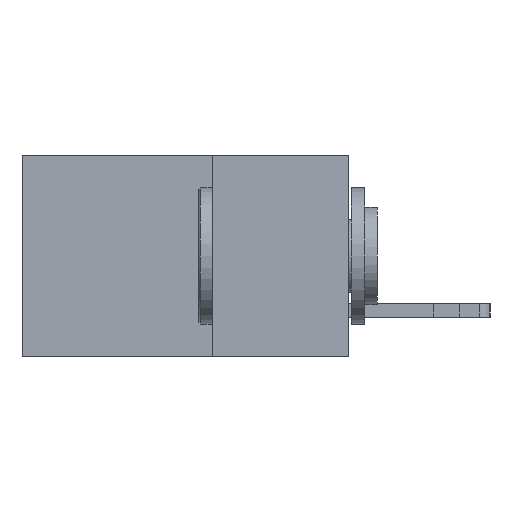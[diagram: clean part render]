
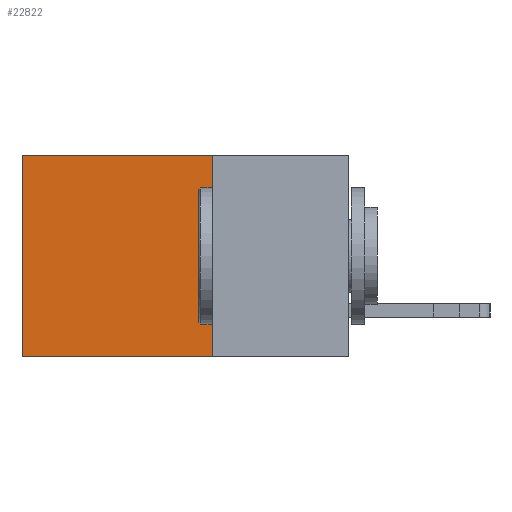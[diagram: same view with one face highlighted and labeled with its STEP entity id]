
A CAD part, left-side view. The second image highlights one B-rep face of the part: STEP entity #22822.
In plain terms, the highlighted planar face has unit normal (-1, 0, 0).
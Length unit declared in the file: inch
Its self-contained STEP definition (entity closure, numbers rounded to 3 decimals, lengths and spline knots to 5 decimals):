
#579 = CARTESIAN_POINT ( 'NONE',  ( 0.298, 0.6, 0. ) ) ;
#1082 = VERTEX_POINT ( 'NONE', #18681 ) ;
#2057 = CARTESIAN_POINT ( 'NONE',  ( 0.298, 0.25, 0. ) ) ;
#2313 = EDGE_CURVE ( 'NONE', #15424, #1082, #12239, .T. ) ;
#3681 = CARTESIAN_POINT ( 'NONE',  ( 0.298, 0.6, 0. ) ) ;
#4080 = DIRECTION ( 'NONE',  ( 1., 0., 0. ) ) ;
#4758 = CARTESIAN_POINT ( 'NONE',  ( 0.298, 0.25, 0. ) ) ;
#5892 = EDGE_CURVE ( 'NONE', #13069, #15424, #20276, .T. ) ;
#6371 = ORIENTED_EDGE ( 'NONE', *, *, #23649, .T. ) ;
#7749 = CARTESIAN_POINT ( 'NONE',  ( 0.298, 0.25, 0. ) ) ;
#8494 = PLANE ( 'NONE',  #19968 ) ;
#8585 = LINE ( 'NONE', #579, #13806 ) ;
#9288 = FACE_OUTER_BOUND ( 'NONE', #9554, .T. ) ;
#9554 = EDGE_LOOP ( 'NONE', ( #6371, #21879, #18293, #24263 ) ) ;
#10781 = DIRECTION ( 'NONE',  ( 0., 0., -1. ) ) ;
#12239 = LINE ( 'NONE', #19379, #17612 ) ;
#13069 = VERTEX_POINT ( 'NONE', #7749 ) ;
#13159 = VECTOR ( 'NONE', #19014, 39.37008 ) ;
#13806 = VECTOR ( 'NONE', #10781, 39.37008 ) ;
#14949 = VECTOR ( 'NONE', #18782, 39.37008 ) ;
#15424 = VERTEX_POINT ( 'NONE', #18578 ) ;
#17612 = VECTOR ( 'NONE', #19561, 39.37008 ) ;
#17864 = LINE ( 'NONE', #4758, #13159 ) ;
#18293 = ORIENTED_EDGE ( 'NONE', *, *, #5892, .F. ) ;
#18349 = DIRECTION ( 'NONE',  ( 0., 0., -1. ) ) ;
#18578 = CARTESIAN_POINT ( 'NONE',  ( 0.298, 0.25, -0.37 ) ) ;
#18681 = CARTESIAN_POINT ( 'NONE',  ( 0.298, 0.6, -0.37 ) ) ;
#18782 = DIRECTION ( 'NONE',  ( 0., 0., -1. ) ) ;
#19014 = DIRECTION ( 'NONE',  ( 0., 1., 0. ) ) ;
#19379 = CARTESIAN_POINT ( 'NONE',  ( 0.298, 0.25, -0.37 ) ) ;
#19561 = DIRECTION ( 'NONE',  ( 0., 1., 0. ) ) ;
#19968 = AXIS2_PLACEMENT_3D ( 'NONE', #2057, #4080, #18349 ) ;
#20276 = LINE ( 'NONE', #20963, #14949 ) ;
#20963 = CARTESIAN_POINT ( 'NONE',  ( 0.298, 0.25, 0. ) ) ;
#21879 = ORIENTED_EDGE ( 'NONE', *, *, #2313, .F. ) ;
#22481 = VERTEX_POINT ( 'NONE', #3681 ) ;
#22822 = ADVANCED_FACE ( 'NONE', ( #9288 ), #8494, .F. ) ;
#23649 = EDGE_CURVE ( 'NONE', #22481, #1082, #8585, .T. ) ;
#23682 = EDGE_CURVE ( 'NONE', #13069, #22481, #17864, .T. ) ;
#24263 = ORIENTED_EDGE ( 'NONE', *, *, #23682, .T. ) ;
